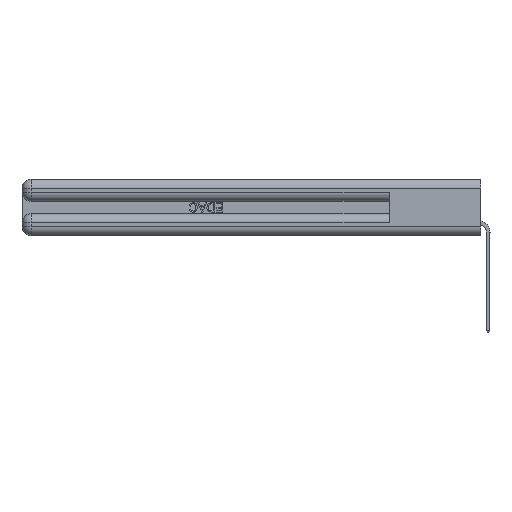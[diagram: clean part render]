
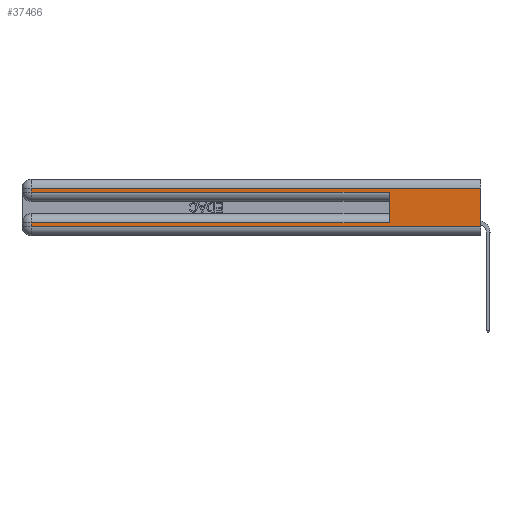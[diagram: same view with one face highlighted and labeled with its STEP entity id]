
A CAD part, left-side view. The second image highlights one B-rep face of the part: STEP entity #37466.
In plain terms, the highlighted planar face has unit normal (-1, 0, 0).
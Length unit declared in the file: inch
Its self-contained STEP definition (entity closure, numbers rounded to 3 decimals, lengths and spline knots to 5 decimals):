
#64 = DIRECTION ( 'NONE',  ( 0., -1., 0. ) ) ;
#392 = VERTEX_POINT ( 'NONE', #45416 ) ;
#1143 = VECTOR ( 'NONE', #19719, 39.37008 ) ;
#1905 = EDGE_CURVE ( 'NONE', #43131, #10165, #12604, .T. ) ;
#2185 = VERTEX_POINT ( 'NONE', #7667 ) ;
#2198 = CARTESIAN_POINT ( 'NONE',  ( 0., 0.6, 0.145 ) ) ;
#2916 = VERTEX_POINT ( 'NONE', #14659 ) ;
#3512 = DIRECTION ( 'NONE',  ( 1., 0., 0. ) ) ;
#5859 = CARTESIAN_POINT ( 'NONE',  ( 0., 0., 0.37 ) ) ;
#5887 = LINE ( 'NONE', #35091, #11909 ) ;
#5925 = VECTOR ( 'NONE', #36895, 39.37008 ) ;
#7667 = CARTESIAN_POINT ( 'NONE',  ( 0., 0., 0.31 ) ) ;
#8132 = CARTESIAN_POINT ( 'NONE',  ( 0., 2.94, 0.37 ) ) ;
#9487 = ORIENTED_EDGE ( 'NONE', *, *, #24805, .T. ) ;
#9894 = CARTESIAN_POINT ( 'NONE',  ( 0., 0., 0.31 ) ) ;
#10165 = VERTEX_POINT ( 'NONE', #44410 ) ;
#10219 = EDGE_CURVE ( 'NONE', #2185, #29383, #11359, .T. ) ;
#11078 = CARTESIAN_POINT ( 'NONE',  ( 0., 2.94, 0.31 ) ) ;
#11143 = CARTESIAN_POINT ( 'NONE',  ( 0., 0., 0.285 ) ) ;
#11248 = DIRECTION ( 'NONE',  ( 0., 0., -1. ) ) ;
#11359 = LINE ( 'NONE', #9894, #5925 ) ;
#11909 = VECTOR ( 'NONE', #19741, 39.37008 ) ;
#12604 = LINE ( 'NONE', #8132, #1143 ) ;
#12709 = EDGE_LOOP ( 'NONE', ( #15967, #15014, #9487, #22595, #24340, #42005, #35035, #16470 ) ) ;
#13003 = VECTOR ( 'NONE', #42157, 39.37008 ) ;
#13469 = DIRECTION ( 'NONE',  ( 0., 0., 1. ) ) ;
#14659 = CARTESIAN_POINT ( 'NONE',  ( 0., 0., 0.06 ) ) ;
#15014 = ORIENTED_EDGE ( 'NONE', *, *, #10219, .T. ) ;
#15967 = ORIENTED_EDGE ( 'NONE', *, *, #37663, .F. ) ;
#15984 = VECTOR ( 'NONE', #64, 39.37008 ) ;
#16470 = ORIENTED_EDGE ( 'NONE', *, *, #35319, .T. ) ;
#17288 = PLANE ( 'NONE',  #47059 ) ;
#18741 = CARTESIAN_POINT ( 'NONE',  ( 0., 0., 0.085 ) ) ;
#19719 = DIRECTION ( 'NONE',  ( 0., 0., -1. ) ) ;
#19741 = DIRECTION ( 'NONE',  ( 0., 0., -1. ) ) ;
#20152 = LINE ( 'NONE', #18741, #25631 ) ;
#22489 = DIRECTION ( 'NONE',  ( 0., 1., 0. ) ) ;
#22595 = ORIENTED_EDGE ( 'NONE', *, *, #35112, .T. ) ;
#23087 = CARTESIAN_POINT ( 'NONE',  ( 0., 0., 0.06 ) ) ;
#24340 = ORIENTED_EDGE ( 'NONE', *, *, #43601, .F. ) ;
#24805 = EDGE_CURVE ( 'NONE', #29383, #392, #5887, .T. ) ;
#25631 = VECTOR ( 'NONE', #22489, 39.37008 ) ;
#29383 = VERTEX_POINT ( 'NONE', #11078 ) ;
#30767 = DIRECTION ( 'NONE',  ( 0., 0., -1. ) ) ;
#32337 = CARTESIAN_POINT ( 'NONE',  ( 0., 0.6, 0.085 ) ) ;
#32669 = VECTOR ( 'NONE', #30767, 39.37008 ) ;
#33543 = VERTEX_POINT ( 'NONE', #32337 ) ;
#35035 = ORIENTED_EDGE ( 'NONE', *, *, #1905, .T. ) ;
#35091 = CARTESIAN_POINT ( 'NONE',  ( 0., 2.94, 0.37 ) ) ;
#35112 = EDGE_CURVE ( 'NONE', #392, #47122, #43733, .T. ) ;
#35319 = EDGE_CURVE ( 'NONE', #10165, #2916, #38360, .T. ) ;
#36319 = LINE ( 'NONE', #49808, #32669 ) ;
#36895 = DIRECTION ( 'NONE',  ( 0., 1., 0. ) ) ;
#37466 = ADVANCED_FACE ( 'NONE', ( #45485 ), #17288, .F. ) ;
#37663 = EDGE_CURVE ( 'NONE', #2185, #2916, #36319, .T. ) ;
#38360 = LINE ( 'NONE', #23087, #15984 ) ;
#38507 = VECTOR ( 'NONE', #13469, 39.37008 ) ;
#39782 = LINE ( 'NONE', #2198, #38507 ) ;
#40708 = EDGE_CURVE ( 'NONE', #33543, #43131, #20152, .T. ) ;
#41876 = CARTESIAN_POINT ( 'NONE',  ( 0., 2.94, 0.085 ) ) ;
#42005 = ORIENTED_EDGE ( 'NONE', *, *, #40708, .T. ) ;
#42157 = DIRECTION ( 'NONE',  ( 0., -1., 0. ) ) ;
#43131 = VERTEX_POINT ( 'NONE', #41876 ) ;
#43601 = EDGE_CURVE ( 'NONE', #33543, #47122, #39782, .T. ) ;
#43733 = LINE ( 'NONE', #11143, #13003 ) ;
#44410 = CARTESIAN_POINT ( 'NONE',  ( 0., 2.94, 0.06 ) ) ;
#45416 = CARTESIAN_POINT ( 'NONE',  ( 0., 2.94, 0.285 ) ) ;
#45485 = FACE_OUTER_BOUND ( 'NONE', #12709, .T. ) ;
#47059 = AXIS2_PLACEMENT_3D ( 'NONE', #5859, #3512, #11248 ) ;
#47122 = VERTEX_POINT ( 'NONE', #47248 ) ;
#47248 = CARTESIAN_POINT ( 'NONE',  ( 0., 0.6, 0.285 ) ) ;
#49808 = CARTESIAN_POINT ( 'NONE',  ( 0., 0., 0.37 ) ) ;
